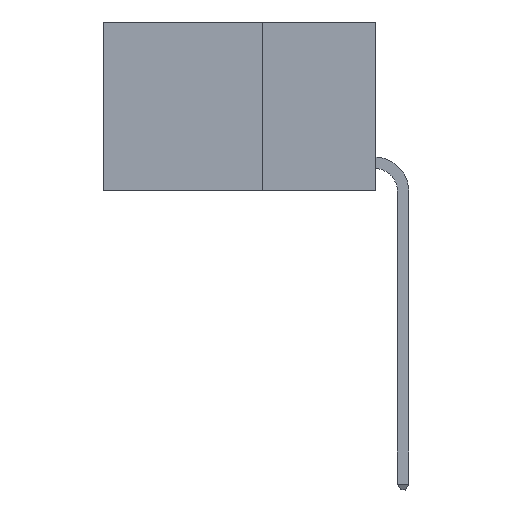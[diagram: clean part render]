
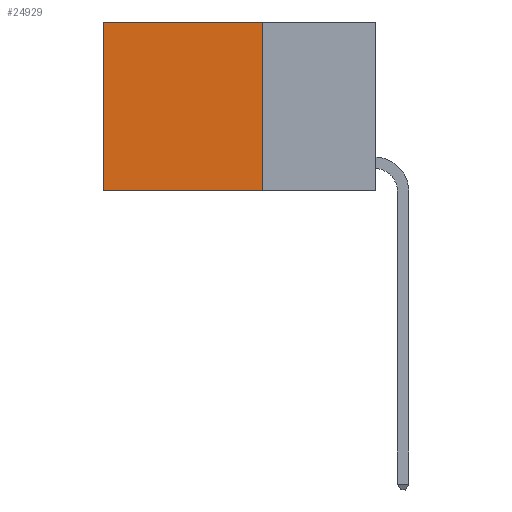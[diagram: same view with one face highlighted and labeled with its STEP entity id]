
A CAD part, left-side view. The second image highlights one B-rep face of the part: STEP entity #24929.
In plain terms, the highlighted planar face has unit normal (-1, 0, 0).
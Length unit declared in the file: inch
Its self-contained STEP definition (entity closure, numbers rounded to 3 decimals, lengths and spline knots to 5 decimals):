
#1926 = DIRECTION ( 'NONE',  ( 0., 0., -1. ) ) ;
#2096 = ORIENTED_EDGE ( 'NONE', *, *, #25719, .F. ) ;
#2310 = EDGE_LOOP ( 'NONE', ( #15530, #2096, #18620, #22701 ) ) ;
#2491 = VERTEX_POINT ( 'NONE', #26640 ) ;
#3203 = VECTOR ( 'NONE', #21418, 39.37008 ) ;
#3673 = CARTESIAN_POINT ( 'NONE',  ( 0.2625, 0.25, 0. ) ) ;
#4372 = CARTESIAN_POINT ( 'NONE',  ( 0.2625, 0.25, -0.37 ) ) ;
#5711 = FACE_OUTER_BOUND ( 'NONE', #2310, .T. ) ;
#5765 = DIRECTION ( 'NONE',  ( 0., 1., 0. ) ) ;
#7236 = CARTESIAN_POINT ( 'NONE',  ( 0.2625, 0.6, 0. ) ) ;
#8059 = LINE ( 'NONE', #7236, #3203 ) ;
#8110 = CARTESIAN_POINT ( 'NONE',  ( 0.2625, 0.25, 0. ) ) ;
#8841 = AXIS2_PLACEMENT_3D ( 'NONE', #8110, #14262, #1926 ) ;
#9016 = EDGE_CURVE ( 'NONE', #20816, #9484, #13116, .T. ) ;
#9484 = VERTEX_POINT ( 'NONE', #22285 ) ;
#10178 = PLANE ( 'NONE',  #8841 ) ;
#10595 = DIRECTION ( 'NONE',  ( 0., 0., -1. ) ) ;
#13116 = LINE ( 'NONE', #22854, #17888 ) ;
#13341 = LINE ( 'NONE', #3673, #23544 ) ;
#13381 = LINE ( 'NONE', #4372, #14032 ) ;
#14032 = VECTOR ( 'NONE', #24766, 39.37008 ) ;
#14262 = DIRECTION ( 'NONE',  ( 1., 0., 0. ) ) ;
#15530 = ORIENTED_EDGE ( 'NONE', *, *, #21569, .T. ) ;
#17888 = VECTOR ( 'NONE', #10595, 39.37008 ) ;
#18620 = ORIENTED_EDGE ( 'NONE', *, *, #9016, .F. ) ;
#20816 = VERTEX_POINT ( 'NONE', #23673 ) ;
#21418 = DIRECTION ( 'NONE',  ( 0., 0., -1. ) ) ;
#21569 = EDGE_CURVE ( 'NONE', #2491, #21784, #8059, .T. ) ;
#21784 = VERTEX_POINT ( 'NONE', #22075 ) ;
#22075 = CARTESIAN_POINT ( 'NONE',  ( 0.2625, 0.6, -0.37 ) ) ;
#22285 = CARTESIAN_POINT ( 'NONE',  ( 0.2625, 0.25, -0.37 ) ) ;
#22701 = ORIENTED_EDGE ( 'NONE', *, *, #24297, .T. ) ;
#22854 = CARTESIAN_POINT ( 'NONE',  ( 0.2625, 0.25, 0. ) ) ;
#23544 = VECTOR ( 'NONE', #5765, 39.37008 ) ;
#23673 = CARTESIAN_POINT ( 'NONE',  ( 0.2625, 0.25, 0. ) ) ;
#24297 = EDGE_CURVE ( 'NONE', #20816, #2491, #13341, .T. ) ;
#24766 = DIRECTION ( 'NONE',  ( 0., 1., 0. ) ) ;
#24929 = ADVANCED_FACE ( 'NONE', ( #5711 ), #10178, .F. ) ;
#25719 = EDGE_CURVE ( 'NONE', #9484, #21784, #13381, .T. ) ;
#26640 = CARTESIAN_POINT ( 'NONE',  ( 0.2625, 0.6, 0. ) ) ;
